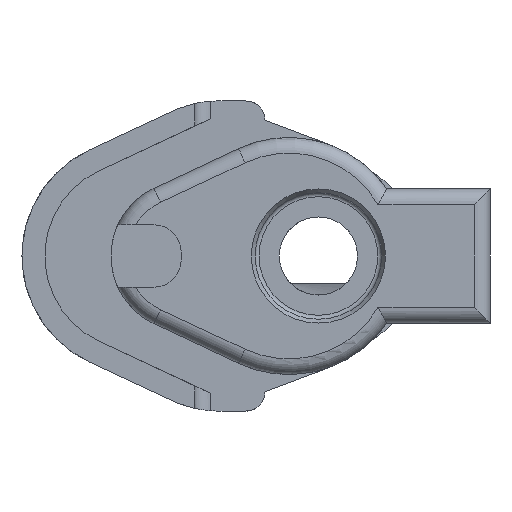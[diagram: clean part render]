
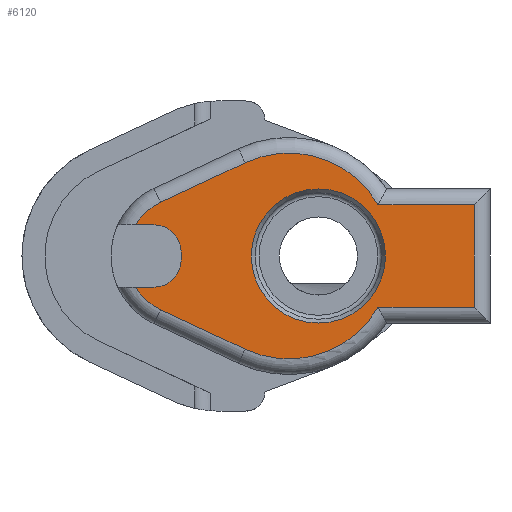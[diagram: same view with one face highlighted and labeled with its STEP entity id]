
A CAD part, left-side view. The second image highlights one B-rep face of the part: STEP entity #6120.
In plain terms, the highlighted planar face has unit normal (-1, 0, 0).
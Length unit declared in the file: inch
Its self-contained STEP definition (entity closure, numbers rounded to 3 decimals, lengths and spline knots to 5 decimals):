
#32=FACE_BOUND('',#1814,.T.);
#167=PLANE('',#6816);
#508=LINE('',#13928,#870);
#509=LINE('',#13942,#871);
#513=LINE('',#13962,#875);
#517=LINE('',#13983,#879);
#518=LINE('',#13987,#880);
#519=LINE('',#13989,#881);
#520=LINE('',#13991,#882);
#521=LINE('',#13994,#883);
#870=VECTOR('',#8428,0.3937);
#871=VECTOR('',#8431,0.3937);
#875=VECTOR('',#8441,0.3937);
#879=VECTOR('',#8469,0.3937);
#880=VECTOR('',#8472,0.3937);
#881=VECTOR('',#8473,0.3937);
#882=VECTOR('',#8474,0.3937);
#883=VECTOR('',#8477,0.3937);
#1433=FACE_OUTER_BOUND('',#1813,.T.);
#1813=EDGE_LOOP('',(#5522,#5523,#5524,#5525,#5526,#5527,#5528,#5529,#5530,
#5531,#5532,#5533,#5534,#5535));
#1814=EDGE_LOOP('',(#5536));
#2173=CIRCLE('',#6803,0.175);
#2174=CIRCLE('',#6806,0.175);
#2178=CIRCLE('',#6812,0.38);
#2179=CIRCLE('',#6814,0.38);
#2181=CIRCLE('',#6817,0.66);
#2182=CIRCLE('',#6818,0.66);
#2183=CIRCLE('',#6819,0.43);
#2897=VERTEX_POINT('',#13925);
#2898=VERTEX_POINT('',#13927);
#2899=VERTEX_POINT('',#13940);
#2900=VERTEX_POINT('',#13941);
#2902=VERTEX_POINT('',#13950);
#2903=VERTEX_POINT('',#13961);
#2906=VERTEX_POINT('',#13974);
#2907=VERTEX_POINT('',#13978);
#2908=VERTEX_POINT('',#13982);
#2909=VERTEX_POINT('',#13984);
#2910=VERTEX_POINT('',#13986);
#2911=VERTEX_POINT('',#13988);
#2912=VERTEX_POINT('',#13990);
#2913=VERTEX_POINT('',#13992);
#2914=VERTEX_POINT('',#13995);
#3787=EDGE_CURVE('',#2898,#2897,#508,.T.);
#3789=EDGE_CURVE('',#2899,#2900,#509,.T.);
#3792=EDGE_CURVE('',#2897,#2899,#2173,.T.);
#3795=EDGE_CURVE('',#2903,#2902,#513,.T.);
#3797=EDGE_CURVE('',#2900,#2903,#2174,.T.);
#3803=EDGE_CURVE('',#2906,#2902,#2178,.T.);
#3804=EDGE_CURVE('',#2898,#2907,#2179,.T.);
#3806=EDGE_CURVE('',#2908,#2906,#517,.T.);
#3807=EDGE_CURVE('',#2909,#2908,#2181,.T.);
#3808=EDGE_CURVE('',#2910,#2909,#518,.T.);
#3809=EDGE_CURVE('',#2911,#2910,#519,.T.);
#3810=EDGE_CURVE('',#2912,#2911,#520,.T.);
#3811=EDGE_CURVE('',#2913,#2912,#2182,.T.);
#3812=EDGE_CURVE('',#2907,#2913,#521,.T.);
#3813=EDGE_CURVE('',#2914,#2914,#2183,.T.);
#5522=ORIENTED_EDGE('',*,*,#3806,.F.);
#5523=ORIENTED_EDGE('',*,*,#3807,.F.);
#5524=ORIENTED_EDGE('',*,*,#3808,.F.);
#5525=ORIENTED_EDGE('',*,*,#3809,.F.);
#5526=ORIENTED_EDGE('',*,*,#3810,.F.);
#5527=ORIENTED_EDGE('',*,*,#3811,.F.);
#5528=ORIENTED_EDGE('',*,*,#3812,.F.);
#5529=ORIENTED_EDGE('',*,*,#3804,.F.);
#5530=ORIENTED_EDGE('',*,*,#3787,.T.);
#5531=ORIENTED_EDGE('',*,*,#3792,.T.);
#5532=ORIENTED_EDGE('',*,*,#3789,.T.);
#5533=ORIENTED_EDGE('',*,*,#3797,.T.);
#5534=ORIENTED_EDGE('',*,*,#3795,.T.);
#5535=ORIENTED_EDGE('',*,*,#3803,.F.);
#5536=ORIENTED_EDGE('',*,*,#3813,.F.);
#6120=ADVANCED_FACE('',(#1433,#32),#167,.T.);
#6803=AXIS2_PLACEMENT_3D('',#13946,#8436,#8437);
#6806=AXIS2_PLACEMENT_3D('',#13965,#8445,#8446);
#6812=AXIS2_PLACEMENT_3D('',#13976,#8459,#8460);
#6814=AXIS2_PLACEMENT_3D('',#13979,#8463,#8464);
#6816=AXIS2_PLACEMENT_3D('',#13981,#8467,#8468);
#6817=AXIS2_PLACEMENT_3D('',#13985,#8470,#8471);
#6818=AXIS2_PLACEMENT_3D('',#13993,#8475,#8476);
#6819=AXIS2_PLACEMENT_3D('',#13996,#8478,#8479);
#8428=DIRECTION('',(0.,-1.,0.));
#8431=DIRECTION('',(0.,0.,-1.));
#8436=DIRECTION('center_axis',(1.,0.,0.));
#8437=DIRECTION('ref_axis',(0.,-1.,0.));
#8441=DIRECTION('',(0.,1.,0.));
#8445=DIRECTION('center_axis',(1.,0.,0.));
#8446=DIRECTION('ref_axis',(0.,0.,-1.));
#8459=DIRECTION('center_axis',(1.,0.,0.));
#8460=DIRECTION('ref_axis',(0.,1.,0.));
#8463=DIRECTION('center_axis',(1.,0.,0.));
#8464=DIRECTION('ref_axis',(0.,1.,0.));
#8467=DIRECTION('center_axis',(-1.,0.,0.));
#8468=DIRECTION('ref_axis',(0.,0.,1.));
#8469=DIRECTION('',(0.,0.906,0.424));
#8470=DIRECTION('center_axis',(1.,0.,0.));
#8471=DIRECTION('ref_axis',(0.,-0.263,-0.965));
#8472=DIRECTION('',(0.,1.,0.));
#8473=DIRECTION('',(0.,0.,-1.));
#8474=DIRECTION('',(0.,-1.,0.));
#8475=DIRECTION('center_axis',(1.,0.,0.));
#8476=DIRECTION('ref_axis',(0.,-0.263,0.965));
#8477=DIRECTION('',(0.,-0.906,0.424));
#8478=DIRECTION('center_axis',(-1.,0.,0.));
#8479=DIRECTION('ref_axis',(0.,0.,1.));
#13925=CARTESIAN_POINT('',(-0.5,0.955,0.2));
#13927=CARTESIAN_POINT('',(-0.5,1.07311,0.2));
#13928=CARTESIAN_POINT('',(-0.5,0.6225,0.2));
#13940=CARTESIAN_POINT('',(-0.5,0.78,0.025));
#13941=CARTESIAN_POINT('',(-0.5,0.78,-0.025));
#13942=CARTESIAN_POINT('',(-0.5,0.78,0.0125));
#13946=CARTESIAN_POINT('Origin',(-0.5,0.955,0.025));
#13950=CARTESIAN_POINT('',(-0.5,1.07311,-0.2));
#13961=CARTESIAN_POINT('',(-0.5,0.955,-0.2));
#13962=CARTESIAN_POINT('',(-0.5,0.485,-0.2));
#13965=CARTESIAN_POINT('Origin',(-0.5,0.955,-0.025));
#13974=CARTESIAN_POINT('',(-0.5,0.91121,-0.34411));
#13976=CARTESIAN_POINT('Origin',(-0.5,0.75,0.));
#13978=CARTESIAN_POINT('',(-0.5,0.91121,0.34411));
#13979=CARTESIAN_POINT('Origin',(-0.5,0.75,0.));
#13981=CARTESIAN_POINT('Origin',(-0.5,0.015,0.));
#13982=CARTESIAN_POINT('',(-0.5,0.37,-0.59766));
#13983=CARTESIAN_POINT('',(-0.5,0.60986,-0.48529));
#13984=CARTESIAN_POINT('',(-0.5,-0.48158,-0.33));
#13985=CARTESIAN_POINT('Origin',(-0.5,0.09,0.));
#13986=CARTESIAN_POINT('',(-0.5,-1.1,-0.33));
#13987=CARTESIAN_POINT('',(-0.5,-0.26083,-0.33));
#13988=CARTESIAN_POINT('',(-0.5,-1.1,0.33));
#13989=CARTESIAN_POINT('',(-0.5,-1.1,-0.215));
#13990=CARTESIAN_POINT('',(-0.5,-0.48158,0.33));
#13991=CARTESIAN_POINT('',(-0.5,-0.5925,0.33));
#13992=CARTESIAN_POINT('',(-0.5,0.37,0.59766));
#13993=CARTESIAN_POINT('Origin',(-0.5,0.09,0.));
#13994=CARTESIAN_POINT('',(-0.5,0.33925,0.61207));
#13995=CARTESIAN_POINT('',(-0.5,-0.1,-0.43));
#13996=CARTESIAN_POINT('Origin',(-0.5,-0.1,0.));
